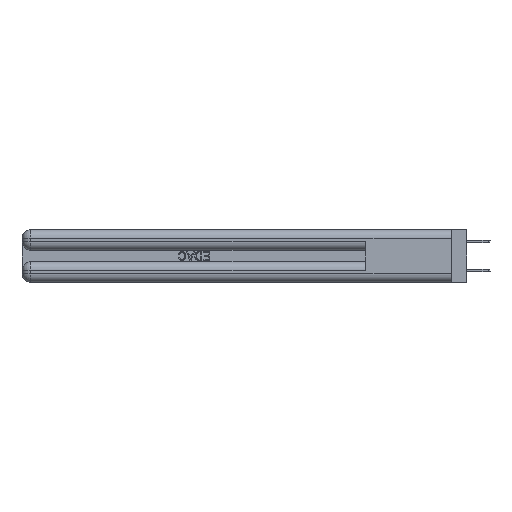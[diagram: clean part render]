
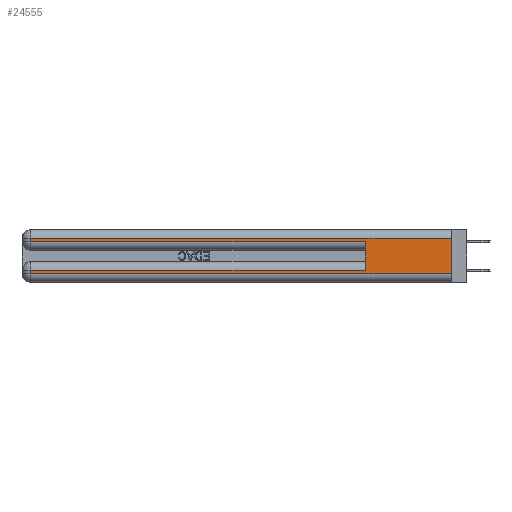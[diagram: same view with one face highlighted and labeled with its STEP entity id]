
A CAD part, left-side view. The second image highlights one B-rep face of the part: STEP entity #24555.
In plain terms, the highlighted planar face has unit normal (-1, 0, 0).
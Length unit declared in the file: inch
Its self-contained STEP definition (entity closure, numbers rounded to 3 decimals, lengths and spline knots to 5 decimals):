
#253 = VECTOR ( 'NONE', #11918, 39.37008 ) ;
#664 = DIRECTION ( 'NONE',  ( 1., 0., 0. ) ) ;
#1157 = EDGE_LOOP ( 'NONE', ( #34008, #27737, #12156, #21417, #5763, #30623, #7732, #18002 ) ) ;
#1259 = LINE ( 'NONE', #36714, #253 ) ;
#1582 = EDGE_CURVE ( 'NONE', #26771, #37510, #18266, .T. ) ;
#2220 = VECTOR ( 'NONE', #12848, 39.37008 ) ;
#2718 = LINE ( 'NONE', #10855, #26670 ) ;
#4247 = EDGE_CURVE ( 'NONE', #32584, #37510, #32694, .T. ) ;
#4678 = CARTESIAN_POINT ( 'NONE',  ( 0., 0., 0.285 ) ) ;
#5418 = VECTOR ( 'NONE', #19212, 39.37008 ) ;
#5763 = ORIENTED_EDGE ( 'NONE', *, *, #1582, .F. ) ;
#6287 = FACE_OUTER_BOUND ( 'NONE', #1157, .T. ) ;
#7732 = ORIENTED_EDGE ( 'NONE', *, *, #27982, .T. ) ;
#8307 = EDGE_CURVE ( 'NONE', #39442, #26176, #2718, .T. ) ;
#9613 = LINE ( 'NONE', #34570, #2220 ) ;
#10855 = CARTESIAN_POINT ( 'NONE',  ( 0., 0., 0.31 ) ) ;
#10991 = DIRECTION ( 'NONE',  ( 0., 1., 0. ) ) ;
#11842 = CARTESIAN_POINT ( 'NONE',  ( 0., 0.6, 0.145 ) ) ;
#11918 = DIRECTION ( 'NONE',  ( 0., -1., 0. ) ) ;
#12156 = ORIENTED_EDGE ( 'NONE', *, *, #33796, .T. ) ;
#12848 = DIRECTION ( 'NONE',  ( 0., 0., -1. ) ) ;
#13090 = LINE ( 'NONE', #17403, #28667 ) ;
#13174 = PLANE ( 'NONE',  #30821 ) ;
#14026 = VECTOR ( 'NONE', #35838, 39.37008 ) ;
#14300 = DIRECTION ( 'NONE',  ( 0., 0., -1. ) ) ;
#14590 = CARTESIAN_POINT ( 'NONE',  ( 0., 2.94, 0.31 ) ) ;
#16538 = CARTESIAN_POINT ( 'NONE',  ( 0., 0., 0.31 ) ) ;
#17403 = CARTESIAN_POINT ( 'NONE',  ( 0., 2.94, 0.37 ) ) ;
#17975 = CARTESIAN_POINT ( 'NONE',  ( 0., 2.94, 0.06 ) ) ;
#18002 = ORIENTED_EDGE ( 'NONE', *, *, #25583, .T. ) ;
#18099 = CARTESIAN_POINT ( 'NONE',  ( 0., 2.94, 0.085 ) ) ;
#18266 = LINE ( 'NONE', #11842, #27534 ) ;
#18968 = CARTESIAN_POINT ( 'NONE',  ( 0., 0., 0.06 ) ) ;
#19212 = DIRECTION ( 'NONE',  ( 0., 1., 0. ) ) ;
#19432 = CARTESIAN_POINT ( 'NONE',  ( 0., 0., 0.37 ) ) ;
#20133 = CARTESIAN_POINT ( 'NONE',  ( 0., 2.94, 0.285 ) ) ;
#21417 = ORIENTED_EDGE ( 'NONE', *, *, #4247, .T. ) ;
#22570 = DIRECTION ( 'NONE',  ( 0., 0., -1. ) ) ;
#23023 = LINE ( 'NONE', #31568, #5418 ) ;
#23415 = DIRECTION ( 'NONE',  ( 0., -1., 0. ) ) ;
#23419 = CARTESIAN_POINT ( 'NONE',  ( 0., 2.94, 0.37 ) ) ;
#24288 = VERTEX_POINT ( 'NONE', #18099 ) ;
#24470 = VECTOR ( 'NONE', #23415, 39.37008 ) ;
#24555 = ADVANCED_FACE ( 'NONE', ( #6287 ), #13174, .F. ) ;
#25583 = EDGE_CURVE ( 'NONE', #36675, #29031, #1259, .T. ) ;
#26059 = CARTESIAN_POINT ( 'NONE',  ( 0., 0.6, 0.285 ) ) ;
#26176 = VERTEX_POINT ( 'NONE', #14590 ) ;
#26670 = VECTOR ( 'NONE', #10991, 39.37008 ) ;
#26771 = VERTEX_POINT ( 'NONE', #38896 ) ;
#27534 = VECTOR ( 'NONE', #30444, 39.37008 ) ;
#27737 = ORIENTED_EDGE ( 'NONE', *, *, #8307, .T. ) ;
#27982 = EDGE_CURVE ( 'NONE', #24288, #36675, #31505, .T. ) ;
#28667 = VECTOR ( 'NONE', #14300, 39.37008 ) ;
#29031 = VERTEX_POINT ( 'NONE', #18968 ) ;
#29055 = EDGE_CURVE ( 'NONE', #39442, #29031, #9613, .T. ) ;
#30444 = DIRECTION ( 'NONE',  ( 0., 0., 1. ) ) ;
#30623 = ORIENTED_EDGE ( 'NONE', *, *, #31869, .T. ) ;
#30821 = AXIS2_PLACEMENT_3D ( 'NONE', #19432, #664, #22570 ) ;
#31505 = LINE ( 'NONE', #23419, #14026 ) ;
#31568 = CARTESIAN_POINT ( 'NONE',  ( 0., 0., 0.085 ) ) ;
#31869 = EDGE_CURVE ( 'NONE', #26771, #24288, #23023, .T. ) ;
#32584 = VERTEX_POINT ( 'NONE', #20133 ) ;
#32694 = LINE ( 'NONE', #4678, #24470 ) ;
#33796 = EDGE_CURVE ( 'NONE', #26176, #32584, #13090, .T. ) ;
#34008 = ORIENTED_EDGE ( 'NONE', *, *, #29055, .F. ) ;
#34570 = CARTESIAN_POINT ( 'NONE',  ( 0., 0., 0.37 ) ) ;
#35838 = DIRECTION ( 'NONE',  ( 0., 0., -1. ) ) ;
#36675 = VERTEX_POINT ( 'NONE', #17975 ) ;
#36714 = CARTESIAN_POINT ( 'NONE',  ( 0., 0., 0.06 ) ) ;
#37510 = VERTEX_POINT ( 'NONE', #26059 ) ;
#38896 = CARTESIAN_POINT ( 'NONE',  ( 0., 0.6, 0.085 ) ) ;
#39442 = VERTEX_POINT ( 'NONE', #16538 ) ;
